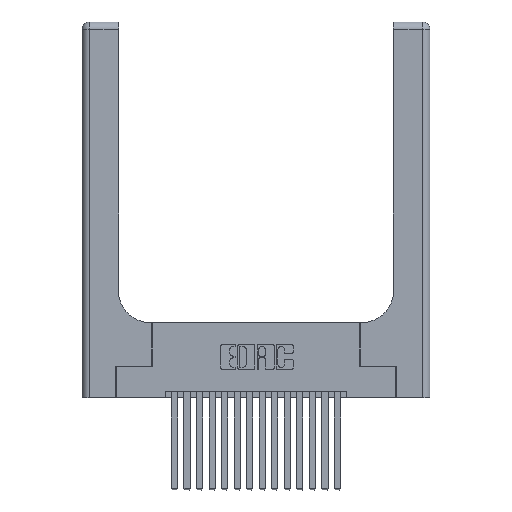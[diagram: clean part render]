
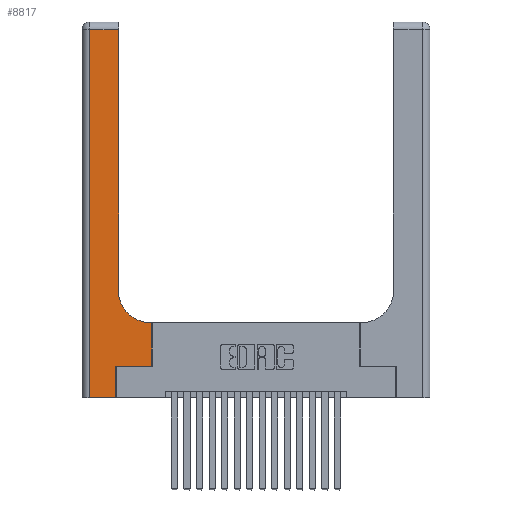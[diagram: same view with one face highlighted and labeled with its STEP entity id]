
A CAD part, top view. The second image highlights one B-rep face of the part: STEP entity #8817.
In plain terms, the highlighted planar face has unit normal (0, 0, 1).
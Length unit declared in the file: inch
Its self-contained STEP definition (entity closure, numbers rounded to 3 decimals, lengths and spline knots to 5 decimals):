
#428 = EDGE_CURVE ( 'NONE', #4170, #8285, #4365, .T. ) ;
#743 = CARTESIAN_POINT ( 'NONE',  ( 0.2915, 2.94, 0.37 ) ) ;
#1447 = DIRECTION ( 'NONE',  ( 0., 1., 0. ) ) ;
#1631 = CARTESIAN_POINT ( 'NONE',  ( 0.269, 0., 0.37 ) ) ;
#1644 = ORIENTED_EDGE ( 'NONE', *, *, #3082, .T. ) ;
#1806 = LINE ( 'NONE', #19643, #13996 ) ;
#1902 = DIRECTION ( 'NONE',  ( 0., -1., 0. ) ) ;
#2006 = EDGE_CURVE ( 'NONE', #15976, #13405, #3018, .T. ) ;
#2679 = CARTESIAN_POINT ( 'NONE',  ( 0.5415, 0.6, 0.37 ) ) ;
#2976 = VECTOR ( 'NONE', #1447, 39.37008 ) ;
#3013 = DIRECTION ( 'NONE',  ( 0., 0., -1. ) ) ;
#3018 = LINE ( 'NONE', #15722, #14652 ) ;
#3082 = EDGE_CURVE ( 'NONE', #9995, #15976, #14614, .T. ) ;
#4070 = VECTOR ( 'NONE', #4813, 39.37008 ) ;
#4170 = VERTEX_POINT ( 'NONE', #743 ) ;
#4365 = LINE ( 'NONE', #16651, #15989 ) ;
#4382 = VERTEX_POINT ( 'NONE', #5521 ) ;
#4733 = CARTESIAN_POINT ( 'NONE',  ( 0.5585, 0.25, 0.37 ) ) ;
#4813 = DIRECTION ( 'NONE',  ( 0., 1., 0. ) ) ;
#5229 = CARTESIAN_POINT ( 'NONE',  ( 0.269, 0.25, 0.37 ) ) ;
#5521 = CARTESIAN_POINT ( 'NONE',  ( 0.06, 0., 0.37 ) ) ;
#5839 = ORIENTED_EDGE ( 'NONE', *, *, #2006, .T. ) ;
#6810 = AXIS2_PLACEMENT_3D ( 'NONE', #12119, #3013, #13629 ) ;
#6977 = AXIS2_PLACEMENT_3D ( 'NONE', #14813, #8832, #19346 ) ;
#7748 = EDGE_CURVE ( 'NONE', #19296, #9995, #1806, .T. ) ;
#8211 = DIRECTION ( 'NONE',  ( -1., 0., 0. ) ) ;
#8285 = VERTEX_POINT ( 'NONE', #19693 ) ;
#8416 = LINE ( 'NONE', #17839, #15956 ) ;
#8447 = ORIENTED_EDGE ( 'NONE', *, *, #13609, .T. ) ;
#8621 = LINE ( 'NONE', #1631, #4070 ) ;
#8766 = PLANE ( 'NONE',  #6977 ) ;
#8817 = ADVANCED_FACE ( 'NONE', ( #18897 ), #8766, .F. ) ;
#8832 = DIRECTION ( 'NONE',  ( 0., 0., -1. ) ) ;
#9136 = DIRECTION ( 'NONE',  ( 1., 0., 0. ) ) ;
#9518 = CARTESIAN_POINT ( 'NONE',  ( 0.06, 3., 0.37 ) ) ;
#9995 = VERTEX_POINT ( 'NONE', #4733 ) ;
#10531 = CARTESIAN_POINT ( 'NONE',  ( 0.2915, 0.85, 0.37 ) ) ;
#11491 = ORIENTED_EDGE ( 'NONE', *, *, #15446, .T. ) ;
#11596 = VERTEX_POINT ( 'NONE', #19187 ) ;
#12119 = CARTESIAN_POINT ( 'NONE',  ( 0.5415, 0.85, 0.37 ) ) ;
#12922 = ORIENTED_EDGE ( 'NONE', *, *, #16103, .T. ) ;
#13020 = EDGE_CURVE ( 'NONE', #11596, #19296, #8621, .T. ) ;
#13040 = CARTESIAN_POINT ( 'NONE',  ( 0.5585, 0.6, 0.37 ) ) ;
#13100 = VECTOR ( 'NONE', #17880, 39.37008 ) ;
#13370 = ORIENTED_EDGE ( 'NONE', *, *, #7748, .T. ) ;
#13405 = VERTEX_POINT ( 'NONE', #2679 ) ;
#13609 = EDGE_CURVE ( 'NONE', #8285, #4382, #18701, .T. ) ;
#13629 = DIRECTION ( 'NONE',  ( 1., 0., 0. ) ) ;
#13996 = VECTOR ( 'NONE', #9136, 39.37008 ) ;
#14330 = ORIENTED_EDGE ( 'NONE', *, *, #15529, .T. ) ;
#14535 = CIRCLE ( 'NONE', #6810, 0.25 ) ;
#14614 = LINE ( 'NONE', #18224, #2976 ) ;
#14652 = VECTOR ( 'NONE', #8211, 39.37008 ) ;
#14813 = CARTESIAN_POINT ( 'NONE',  ( 0., 3., 0.37 ) ) ;
#15446 = EDGE_CURVE ( 'NONE', #16166, #4170, #8416, .T. ) ;
#15529 = EDGE_CURVE ( 'NONE', #13405, #16166, #14535, .T. ) ;
#15722 = CARTESIAN_POINT ( 'NONE',  ( 0.2915, 0.6, 0.37 ) ) ;
#15956 = VECTOR ( 'NONE', #19356, 39.37008 ) ;
#15976 = VERTEX_POINT ( 'NONE', #13040 ) ;
#15982 = ORIENTED_EDGE ( 'NONE', *, *, #428, .T. ) ;
#15989 = VECTOR ( 'NONE', #16455, 39.37008 ) ;
#16103 = EDGE_CURVE ( 'NONE', #4382, #11596, #17097, .T. ) ;
#16166 = VERTEX_POINT ( 'NONE', #10531 ) ;
#16375 = CARTESIAN_POINT ( 'NONE',  ( 0., 0., 0.37 ) ) ;
#16455 = DIRECTION ( 'NONE',  ( -1., 0., 0. ) ) ;
#16651 = CARTESIAN_POINT ( 'NONE',  ( 0., 2.94, 0.37 ) ) ;
#16912 = ORIENTED_EDGE ( 'NONE', *, *, #13020, .T. ) ;
#16955 = EDGE_LOOP ( 'NONE', ( #11491, #15982, #8447, #12922, #16912, #13370, #1644, #5839, #14330 ) ) ;
#17097 = LINE ( 'NONE', #16375, #13100 ) ;
#17757 = VECTOR ( 'NONE', #1902, 39.37008 ) ;
#17839 = CARTESIAN_POINT ( 'NONE',  ( 0.2915, 3., 0.37 ) ) ;
#17880 = DIRECTION ( 'NONE',  ( 1., 0., 0. ) ) ;
#18224 = CARTESIAN_POINT ( 'NONE',  ( 0.5585, 0.25, 0.37 ) ) ;
#18701 = LINE ( 'NONE', #9518, #17757 ) ;
#18897 = FACE_OUTER_BOUND ( 'NONE', #16955, .T. ) ;
#19187 = CARTESIAN_POINT ( 'NONE',  ( 0.269, 0., 0.37 ) ) ;
#19296 = VERTEX_POINT ( 'NONE', #5229 ) ;
#19346 = DIRECTION ( 'NONE',  ( -1., 0., 0. ) ) ;
#19356 = DIRECTION ( 'NONE',  ( 0., 1., 0. ) ) ;
#19643 = CARTESIAN_POINT ( 'NONE',  ( 0.269, 0.25, 0.37 ) ) ;
#19693 = CARTESIAN_POINT ( 'NONE',  ( 0.06, 2.94, 0.37 ) ) ;
